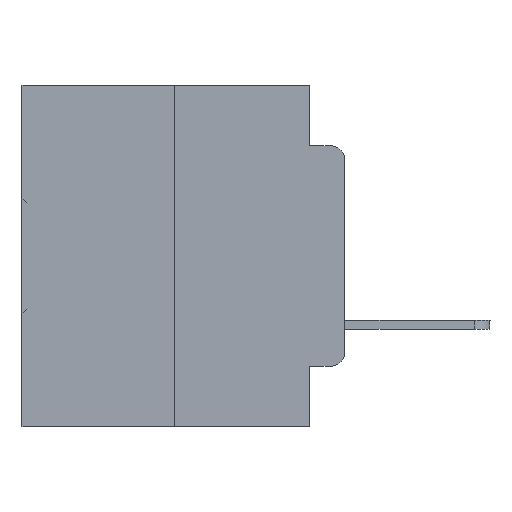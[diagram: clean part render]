
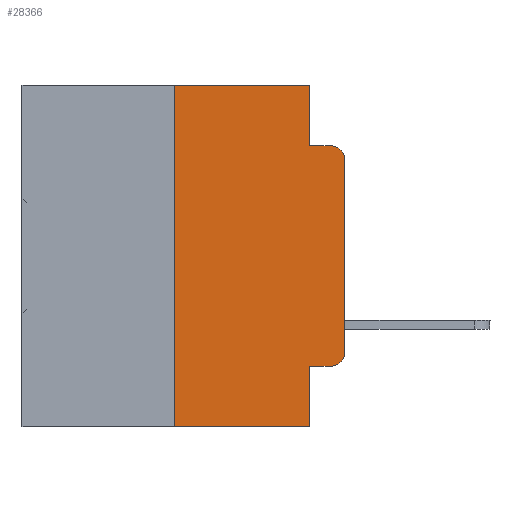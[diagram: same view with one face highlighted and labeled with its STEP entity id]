
A CAD part, left-side view. The second image highlights one B-rep face of the part: STEP entity #28366.
In plain terms, the highlighted planar face has unit normal (-1, 0, 0).
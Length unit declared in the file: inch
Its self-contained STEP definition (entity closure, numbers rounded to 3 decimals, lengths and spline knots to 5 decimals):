
#525 = CARTESIAN_POINT ( 'NONE',  ( 0., 0.051, -0.0885 ) ) ;
#604 = VECTOR ( 'NONE', #26013, 39.37008 ) ;
#816 = DIRECTION ( 'NONE',  ( 0., 0., -1. ) ) ;
#1877 = ORIENTED_EDGE ( 'NONE', *, *, #7540, .T. ) ;
#1881 = DIRECTION ( 'NONE',  ( 1., 0., 0. ) ) ;
#2632 = ORIENTED_EDGE ( 'NONE', *, *, #6649, .T. ) ;
#2976 = ORIENTED_EDGE ( 'NONE', *, *, #22060, .T. ) ;
#3114 = DIRECTION ( 'NONE',  ( -1., 0., 0. ) ) ;
#3157 = CARTESIAN_POINT ( 'NONE',  ( 0., 0., 0. ) ) ;
#3353 = CARTESIAN_POINT ( 'NONE',  ( 0., 0.02, -0.1085 ) ) ;
#3686 = VECTOR ( 'NONE', #26190, 39.37008 ) ;
#5487 = DIRECTION ( 'NONE',  ( 0., 0., -1. ) ) ;
#5861 = CIRCLE ( 'NONE', #33213, 0.02 ) ;
#6225 = LINE ( 'NONE', #3157, #21062 ) ;
#6256 = ORIENTED_EDGE ( 'NONE', *, *, #25945, .F. ) ;
#6649 = EDGE_CURVE ( 'NONE', #31381, #15932, #6225, .T. ) ;
#6900 = DIRECTION ( 'NONE',  ( 0., 0., 1. ) ) ;
#7540 = EDGE_CURVE ( 'NONE', #23116, #9715, #9859, .T. ) ;
#7744 = CARTESIAN_POINT ( 'NONE',  ( 0., 0.473, -0.5 ) ) ;
#8517 = LINE ( 'NONE', #32001, #30805 ) ;
#9206 = EDGE_CURVE ( 'NONE', #29899, #28714, #8517, .T. ) ;
#9567 = EDGE_CURVE ( 'NONE', #25238, #21293, #32859, .T. ) ;
#9715 = VERTEX_POINT ( 'NONE', #18520 ) ;
#9859 = LINE ( 'NONE', #7744, #3686 ) ;
#9963 = CARTESIAN_POINT ( 'NONE',  ( 0., 0.473, 0. ) ) ;
#10436 = CARTESIAN_POINT ( 'NONE',  ( 0., 0.051, -0.4115 ) ) ;
#11295 = CARTESIAN_POINT ( 'NONE',  ( 0., 0.25, 0. ) ) ;
#11682 = CARTESIAN_POINT ( 'NONE',  ( 0., 0.051, 0. ) ) ;
#11696 = ORIENTED_EDGE ( 'NONE', *, *, #23559, .F. ) ;
#11995 = VERTEX_POINT ( 'NONE', #10436 ) ;
#12857 = PLANE ( 'NONE',  #18722 ) ;
#13080 = EDGE_CURVE ( 'NONE', #11995, #21791, #17338, .T. ) ;
#13281 = ORIENTED_EDGE ( 'NONE', *, *, #32147, .T. ) ;
#14199 = CARTESIAN_POINT ( 'NONE',  ( 0., 0.051, -0.4115 ) ) ;
#15374 = CARTESIAN_POINT ( 'NONE',  ( 0., 0.051, 0. ) ) ;
#15932 = VERTEX_POINT ( 'NONE', #22835 ) ;
#16395 = DIRECTION ( 'NONE',  ( 0., -1., 0. ) ) ;
#16819 = LINE ( 'NONE', #20025, #30886 ) ;
#17338 = LINE ( 'NONE', #14199, #29362 ) ;
#17897 = DIRECTION ( 'NONE',  ( 0., 0., -1. ) ) ;
#17969 = CARTESIAN_POINT ( 'NONE',  ( 0., 0.02, -0.4115 ) ) ;
#18065 = ORIENTED_EDGE ( 'NONE', *, *, #26203, .F. ) ;
#18254 = CIRCLE ( 'NONE', #22773, 0.02 ) ;
#18520 = CARTESIAN_POINT ( 'NONE',  ( 0., 0.051, -0.5 ) ) ;
#18557 = VECTOR ( 'NONE', #816, 39.37008 ) ;
#18722 = AXIS2_PLACEMENT_3D ( 'NONE', #9963, #1881, #17897 ) ;
#19823 = ORIENTED_EDGE ( 'NONE', *, *, #9567, .F. ) ;
#20025 = CARTESIAN_POINT ( 'NONE',  ( 0., 0.25, 0. ) ) ;
#20207 = CARTESIAN_POINT ( 'NONE',  ( 0., 0., -0.3915 ) ) ;
#20834 = ORIENTED_EDGE ( 'NONE', *, *, #9206, .F. ) ;
#21062 = VECTOR ( 'NONE', #21609, 39.37008 ) ;
#21293 = VERTEX_POINT ( 'NONE', #15374 ) ;
#21383 = CARTESIAN_POINT ( 'NONE',  ( 0., 0.051, 0. ) ) ;
#21609 = DIRECTION ( 'NONE',  ( 0., 0., 1. ) ) ;
#21791 = VERTEX_POINT ( 'NONE', #17969 ) ;
#22060 = EDGE_CURVE ( 'NONE', #15932, #28714, #18254, .T. ) ;
#22773 = AXIS2_PLACEMENT_3D ( 'NONE', #3353, #32331, #32102 ) ;
#22835 = CARTESIAN_POINT ( 'NONE',  ( 0., 0., -0.1085 ) ) ;
#23116 = VERTEX_POINT ( 'NONE', #27613 ) ;
#23425 = LINE ( 'NONE', #21383, #30458 ) ;
#23559 = EDGE_CURVE ( 'NONE', #21293, #29899, #25969, .T. ) ;
#24223 = CARTESIAN_POINT ( 'NONE',  ( 0., 0.02, -0.3915 ) ) ;
#25238 = VERTEX_POINT ( 'NONE', #11295 ) ;
#25945 = EDGE_CURVE ( 'NONE', #23116, #25238, #16819, .T. ) ;
#25969 = LINE ( 'NONE', #11682, #18557 ) ;
#26013 = DIRECTION ( 'NONE',  ( 0., -1., 0. ) ) ;
#26190 = DIRECTION ( 'NONE',  ( 0., -1., 0. ) ) ;
#26203 = EDGE_CURVE ( 'NONE', #11995, #9715, #23425, .T. ) ;
#27613 = CARTESIAN_POINT ( 'NONE',  ( 0., 0.25, -0.5 ) ) ;
#28366 = ADVANCED_FACE ( 'NONE', ( #33638 ), #12857, .F. ) ;
#28714 = VERTEX_POINT ( 'NONE', #32707 ) ;
#29166 = EDGE_LOOP ( 'NONE', ( #2632, #2976, #20834, #11696, #19823, #6256, #1877, #18065, #33521, #13281 ) ) ;
#29187 = DIRECTION ( 'NONE',  ( 0., 0., -1. ) ) ;
#29362 = VECTOR ( 'NONE', #16395, 39.37008 ) ;
#29899 = VERTEX_POINT ( 'NONE', #525 ) ;
#30458 = VECTOR ( 'NONE', #5487, 39.37008 ) ;
#30805 = VECTOR ( 'NONE', #31392, 39.37008 ) ;
#30886 = VECTOR ( 'NONE', #6900, 39.37008 ) ;
#31381 = VERTEX_POINT ( 'NONE', #20207 ) ;
#31392 = DIRECTION ( 'NONE',  ( 0., -1., 0. ) ) ;
#32001 = CARTESIAN_POINT ( 'NONE',  ( 0., 0.051, -0.0885 ) ) ;
#32102 = DIRECTION ( 'NONE',  ( 0., 0., -1. ) ) ;
#32147 = EDGE_CURVE ( 'NONE', #21791, #31381, #5861, .T. ) ;
#32331 = DIRECTION ( 'NONE',  ( -1., 0., 0. ) ) ;
#32707 = CARTESIAN_POINT ( 'NONE',  ( 0., 0.02, -0.0885 ) ) ;
#32859 = LINE ( 'NONE', #34018, #604 ) ;
#33213 = AXIS2_PLACEMENT_3D ( 'NONE', #24223, #3114, #29187 ) ;
#33521 = ORIENTED_EDGE ( 'NONE', *, *, #13080, .T. ) ;
#33638 = FACE_OUTER_BOUND ( 'NONE', #29166, .T. ) ;
#34018 = CARTESIAN_POINT ( 'NONE',  ( 0., 0.473, 0. ) ) ;
